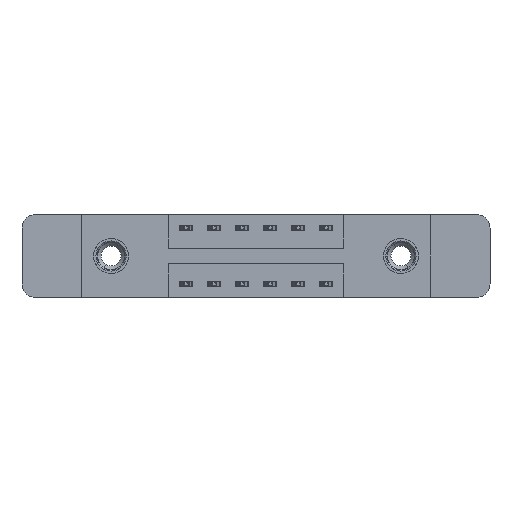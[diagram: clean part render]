
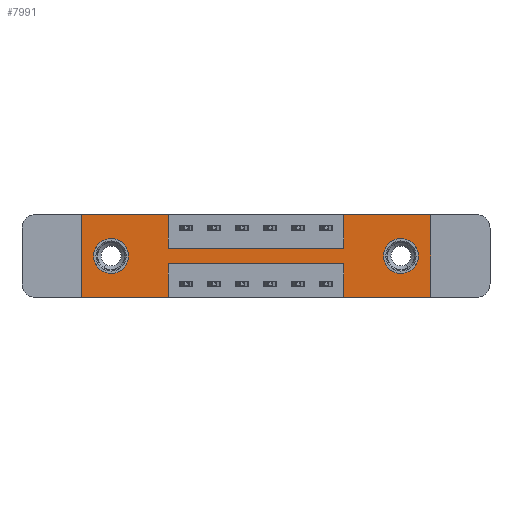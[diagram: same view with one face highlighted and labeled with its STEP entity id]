
A CAD part, front view. The second image highlights one B-rep face of the part: STEP entity #7991.
In plain terms, the highlighted planar face has unit normal (0, -1, 0).
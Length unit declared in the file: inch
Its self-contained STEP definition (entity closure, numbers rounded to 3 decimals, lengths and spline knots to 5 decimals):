
#140 = CARTESIAN_POINT ( 'NONE',  ( 0.3875, 0., 0. ) ) ;
#275 = CARTESIAN_POINT ( 'NONE',  ( 0.1325, 0., -0.185 ) ) ;
#287 = LINE ( 'NONE', #1453, #3701 ) ;
#290 = DIRECTION ( 'NONE',  ( 0., 0., -1. ) ) ;
#521 = CARTESIAN_POINT ( 'NONE',  ( 1.56, 0., 0. ) ) ;
#619 = EDGE_CURVE ( 'NONE', #5092, #2734, #287, .T. ) ;
#631 = ORIENTED_EDGE ( 'NONE', *, *, #1016, .F. ) ;
#634 = CARTESIAN_POINT ( 'NONE',  ( 1.4275, 0., -0.185 ) ) ;
#713 = ORIENTED_EDGE ( 'NONE', *, *, #10029, .F. ) ;
#883 = EDGE_CURVE ( 'NONE', #8422, #3009, #3248, .T. ) ;
#996 = LINE ( 'NONE', #12433, #12143 ) ;
#1016 = EDGE_CURVE ( 'NONE', #2734, #8617, #12821, .T. ) ;
#1023 = EDGE_CURVE ( 'NONE', #5341, #6179, #996, .T. ) ;
#1033 = ORIENTED_EDGE ( 'NONE', *, *, #13043, .F. ) ;
#1095 = CIRCLE ( 'NONE', #5080, 0.078 ) ;
#1132 = DIRECTION ( 'NONE',  ( 0., 0., -1. ) ) ;
#1168 = CARTESIAN_POINT ( 'NONE',  ( 1.1725, 0., -0.37 ) ) ;
#1287 = VERTEX_POINT ( 'NONE', #7413 ) ;
#1291 = CARTESIAN_POINT ( 'NONE',  ( 0., 0., 0. ) ) ;
#1338 = DIRECTION ( 'NONE',  ( 0., 0., 1. ) ) ;
#1352 = CIRCLE ( 'NONE', #12261, 0.078 ) ;
#1378 = ORIENTED_EDGE ( 'NONE', *, *, #2494, .F. ) ;
#1453 = CARTESIAN_POINT ( 'NONE',  ( 0., 0., 0. ) ) ;
#1676 = DIRECTION ( 'NONE',  ( 0., 1., 0. ) ) ;
#1735 = ORIENTED_EDGE ( 'NONE', *, *, #6210, .T. ) ;
#1846 = CARTESIAN_POINT ( 'NONE',  ( 1.56, 0., -0.37 ) ) ;
#1956 = LINE ( 'NONE', #11369, #11376 ) ;
#2000 = LINE ( 'NONE', #3787, #13626 ) ;
#2105 = VERTEX_POINT ( 'NONE', #4366 ) ;
#2384 = DIRECTION ( 'NONE',  ( 0., 0., 1. ) ) ;
#2419 = CARTESIAN_POINT ( 'NONE',  ( 0., 0., -0.37 ) ) ;
#2494 = EDGE_CURVE ( 'NONE', #10658, #5092, #6199, .T. ) ;
#2601 = CIRCLE ( 'NONE', #12430, 0.078 ) ;
#2664 = EDGE_CURVE ( 'NONE', #3009, #8422, #1095, .T. ) ;
#2719 = DIRECTION ( 'NONE',  ( 0., 0., 1. ) ) ;
#2734 = VERTEX_POINT ( 'NONE', #12377 ) ;
#2758 = DIRECTION ( 'NONE',  ( 1., 0., 0. ) ) ;
#2992 = EDGE_LOOP ( 'NONE', ( #4878, #1033, #10724, #13802, #631, #3226, #1378, #8829, #713, #4916, #4737, #3794 ) ) ;
#3009 = VERTEX_POINT ( 'NONE', #9663 ) ;
#3226 = ORIENTED_EDGE ( 'NONE', *, *, #619, .F. ) ;
#3248 = CIRCLE ( 'NONE', #4069, 0.078 ) ;
#3315 = EDGE_CURVE ( 'NONE', #1287, #12833, #1956, .T. ) ;
#3397 = FACE_BOUND ( 'NONE', #9529, .T. ) ;
#3478 = LINE ( 'NONE', #8901, #7713 ) ;
#3511 = EDGE_CURVE ( 'NONE', #12833, #12208, #7718, .T. ) ;
#3642 = VECTOR ( 'NONE', #6650, 39.37008 ) ;
#3652 = VECTOR ( 'NONE', #7849, 39.37008 ) ;
#3701 = VECTOR ( 'NONE', #13264, 39.37008 ) ;
#3787 = CARTESIAN_POINT ( 'NONE',  ( 0.3875, 0., -0.15 ) ) ;
#3794 = ORIENTED_EDGE ( 'NONE', *, *, #3315, .F. ) ;
#3986 = CARTESIAN_POINT ( 'NONE',  ( 1.1725, 0., 0. ) ) ;
#4025 = CARTESIAN_POINT ( 'NONE',  ( 0.3875, 0., -0.22 ) ) ;
#4069 = AXIS2_PLACEMENT_3D ( 'NONE', #13942, #13109, #2384 ) ;
#4241 = VECTOR ( 'NONE', #6726, 39.37008 ) ;
#4364 = CARTESIAN_POINT ( 'NONE',  ( 0.3875, 0., -0.37 ) ) ;
#4366 = CARTESIAN_POINT ( 'NONE',  ( 1.4275, 0., -0.263 ) ) ;
#4369 = PLANE ( 'NONE',  #5547 ) ;
#4458 = CARTESIAN_POINT ( 'NONE',  ( 1.4275, 0., -0.107 ) ) ;
#4737 = ORIENTED_EDGE ( 'NONE', *, *, #3511, .F. ) ;
#4878 = ORIENTED_EDGE ( 'NONE', *, *, #9081, .F. ) ;
#4916 = ORIENTED_EDGE ( 'NONE', *, *, #10249, .F. ) ;
#4923 = EDGE_CURVE ( 'NONE', #2105, #9288, #2601, .T. ) ;
#4930 = CARTESIAN_POINT ( 'NONE',  ( 1.1725, 0., -0.15 ) ) ;
#5080 = AXIS2_PLACEMENT_3D ( 'NONE', #275, #13106, #1338 ) ;
#5092 = VERTEX_POINT ( 'NONE', #8811 ) ;
#5126 = LINE ( 'NONE', #13579, #13727 ) ;
#5341 = VERTEX_POINT ( 'NONE', #1168 ) ;
#5455 = CARTESIAN_POINT ( 'NONE',  ( 0.1325, 0., -0.107 ) ) ;
#5456 = DIRECTION ( 'NONE',  ( 0., -1., 0. ) ) ;
#5547 = AXIS2_PLACEMENT_3D ( 'NONE', #11892, #5456, #1132 ) ;
#6179 = VERTEX_POINT ( 'NONE', #7641 ) ;
#6199 = LINE ( 'NONE', #3986, #11400 ) ;
#6210 = EDGE_CURVE ( 'NONE', #9288, #2105, #1352, .T. ) ;
#6477 = VECTOR ( 'NONE', #8822, 39.37008 ) ;
#6650 = DIRECTION ( 'NONE',  ( 0., 0., 1. ) ) ;
#6726 = DIRECTION ( 'NONE',  ( -1., 0., 0. ) ) ;
#7017 = LINE ( 'NONE', #2419, #6477 ) ;
#7113 = FACE_OUTER_BOUND ( 'NONE', #2992, .T. ) ;
#7150 = VECTOR ( 'NONE', #8091, 39.37008 ) ;
#7252 = DIRECTION ( 'NONE',  ( 0., 0., -1. ) ) ;
#7413 = CARTESIAN_POINT ( 'NONE',  ( 0.3875, 0., -0.37 ) ) ;
#7641 = CARTESIAN_POINT ( 'NONE',  ( 1.1725, 0., -0.22 ) ) ;
#7713 = VECTOR ( 'NONE', #290, 39.37008 ) ;
#7718 = LINE ( 'NONE', #1291, #3642 ) ;
#7735 = DIRECTION ( 'NONE',  ( 0., 0., -1. ) ) ;
#7849 = DIRECTION ( 'NONE',  ( 0., 0., -1. ) ) ;
#7972 = LINE ( 'NONE', #4025, #4241 ) ;
#7991 = ADVANCED_FACE ( 'NONE', ( #12450, #3397, #7113 ), #4369, .T. ) ;
#8000 = CARTESIAN_POINT ( 'NONE',  ( 0.3875, 0., -0.15 ) ) ;
#8091 = DIRECTION ( 'NONE',  ( 0., 0., -1. ) ) ;
#8422 = VERTEX_POINT ( 'NONE', #5455 ) ;
#8546 = EDGE_CURVE ( 'NONE', #12438, #10658, #2000, .T. ) ;
#8617 = VERTEX_POINT ( 'NONE', #1846 ) ;
#8811 = CARTESIAN_POINT ( 'NONE',  ( 1.1725, 0., 0. ) ) ;
#8822 = DIRECTION ( 'NONE',  ( -1., 0., 0. ) ) ;
#8829 = ORIENTED_EDGE ( 'NONE', *, *, #8546, .F. ) ;
#8881 = CARTESIAN_POINT ( 'NONE',  ( 0.3875, 0., -0.22 ) ) ;
#8901 = CARTESIAN_POINT ( 'NONE',  ( 0.3875, 0., 0. ) ) ;
#9081 = EDGE_CURVE ( 'NONE', #9086, #1287, #9566, .T. ) ;
#9086 = VERTEX_POINT ( 'NONE', #8881 ) ;
#9288 = VERTEX_POINT ( 'NONE', #4458 ) ;
#9516 = VERTEX_POINT ( 'NONE', #140 ) ;
#9529 = EDGE_LOOP ( 'NONE', ( #10011, #11932 ) ) ;
#9566 = LINE ( 'NONE', #4364, #3652 ) ;
#9663 = CARTESIAN_POINT ( 'NONE',  ( 0.1325, 0., -0.263 ) ) ;
#9770 = CARTESIAN_POINT ( 'NONE',  ( 1.4275, 0., -0.185 ) ) ;
#10011 = ORIENTED_EDGE ( 'NONE', *, *, #883, .T. ) ;
#10029 = EDGE_CURVE ( 'NONE', #9516, #12438, #3478, .T. ) ;
#10249 = EDGE_CURVE ( 'NONE', #12208, #9516, #5126, .T. ) ;
#10623 = EDGE_LOOP ( 'NONE', ( #1735, #13048 ) ) ;
#10658 = VERTEX_POINT ( 'NONE', #4930 ) ;
#10697 = CARTESIAN_POINT ( 'NONE',  ( 0., 0., 0. ) ) ;
#10724 = ORIENTED_EDGE ( 'NONE', *, *, #1023, .F. ) ;
#10940 = EDGE_CURVE ( 'NONE', #8617, #5341, #7017, .T. ) ;
#11047 = CARTESIAN_POINT ( 'NONE',  ( 0., 0., -0.37 ) ) ;
#11369 = CARTESIAN_POINT ( 'NONE',  ( 0., 0., -0.37 ) ) ;
#11376 = VECTOR ( 'NONE', #13400, 39.37008 ) ;
#11400 = VECTOR ( 'NONE', #11590, 39.37008 ) ;
#11590 = DIRECTION ( 'NONE',  ( 0., 0., 1. ) ) ;
#11892 = CARTESIAN_POINT ( 'NONE',  ( 0., 0., -0.37 ) ) ;
#11932 = ORIENTED_EDGE ( 'NONE', *, *, #2664, .T. ) ;
#12143 = VECTOR ( 'NONE', #2719, 39.37008 ) ;
#12208 = VERTEX_POINT ( 'NONE', #10697 ) ;
#12261 = AXIS2_PLACEMENT_3D ( 'NONE', #9770, #13052, #7735 ) ;
#12377 = CARTESIAN_POINT ( 'NONE',  ( 1.56, 0., 0. ) ) ;
#12430 = AXIS2_PLACEMENT_3D ( 'NONE', #634, #1676, #7252 ) ;
#12433 = CARTESIAN_POINT ( 'NONE',  ( 1.1725, 0., -0.37 ) ) ;
#12438 = VERTEX_POINT ( 'NONE', #8000 ) ;
#12450 = FACE_BOUND ( 'NONE', #10623, .T. ) ;
#12497 = DIRECTION ( 'NONE',  ( 1., 0., 0. ) ) ;
#12821 = LINE ( 'NONE', #521, #7150 ) ;
#12833 = VERTEX_POINT ( 'NONE', #11047 ) ;
#13043 = EDGE_CURVE ( 'NONE', #6179, #9086, #7972, .T. ) ;
#13048 = ORIENTED_EDGE ( 'NONE', *, *, #4923, .T. ) ;
#13052 = DIRECTION ( 'NONE',  ( 0., 1., 0. ) ) ;
#13106 = DIRECTION ( 'NONE',  ( 0., 1., 0. ) ) ;
#13109 = DIRECTION ( 'NONE',  ( 0., 1., 0. ) ) ;
#13264 = DIRECTION ( 'NONE',  ( 1., 0., 0. ) ) ;
#13400 = DIRECTION ( 'NONE',  ( -1., 0., 0. ) ) ;
#13579 = CARTESIAN_POINT ( 'NONE',  ( 0., 0., 0. ) ) ;
#13626 = VECTOR ( 'NONE', #2758, 39.37008 ) ;
#13727 = VECTOR ( 'NONE', #12497, 39.37008 ) ;
#13802 = ORIENTED_EDGE ( 'NONE', *, *, #10940, .F. ) ;
#13942 = CARTESIAN_POINT ( 'NONE',  ( 0.1325, 0., -0.185 ) ) ;
